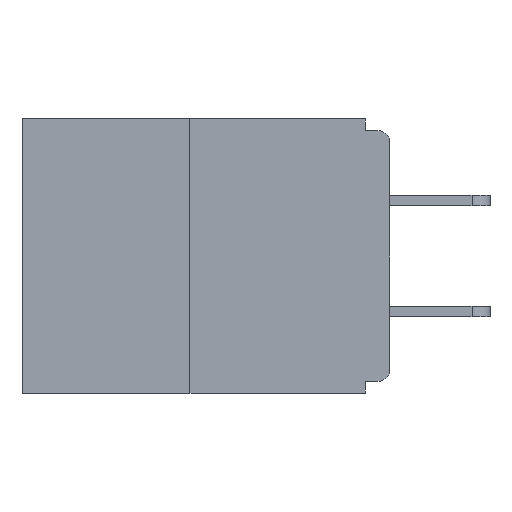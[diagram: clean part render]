
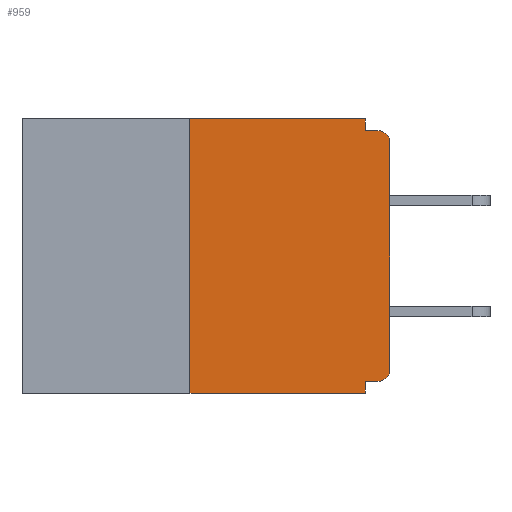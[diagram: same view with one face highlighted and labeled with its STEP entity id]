
A CAD part, left-side view. The second image highlights one B-rep face of the part: STEP entity #959.
In plain terms, the highlighted planar face has unit normal (-1, 0, 0).
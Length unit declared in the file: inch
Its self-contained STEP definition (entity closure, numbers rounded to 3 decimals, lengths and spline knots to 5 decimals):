
#425 = VECTOR ( 'NONE', #7176, 39.37008 ) ;
#959 = ADVANCED_FACE ( 'NONE', ( #2460 ), #17835, .F. ) ;
#1201 = VERTEX_POINT ( 'NONE', #17958 ) ;
#1491 = CARTESIAN_POINT ( 'NONE',  ( 0., 0.031, -0.015 ) ) ;
#1503 = VERTEX_POINT ( 'NONE', #8946 ) ;
#1510 = ORIENTED_EDGE ( 'NONE', *, *, #19461, .F. ) ;
#1680 = LINE ( 'NONE', #15199, #425 ) ;
#2442 = AXIS2_PLACEMENT_3D ( 'NONE', #6521, #6595, #19144 ) ;
#2460 = FACE_OUTER_BOUND ( 'NONE', #2973, .T. ) ;
#2553 = CARTESIAN_POINT ( 'NONE',  ( 0., 0.25, 0. ) ) ;
#2615 = CARTESIAN_POINT ( 'NONE',  ( 0., 0., -0.313 ) ) ;
#2715 = VECTOR ( 'NONE', #12299, 39.37008 ) ;
#2721 = EDGE_CURVE ( 'NONE', #8084, #14545, #8117, .T. ) ;
#2916 = CARTESIAN_POINT ( 'NONE',  ( 0., 0.031, 0. ) ) ;
#2940 = CARTESIAN_POINT ( 'NONE',  ( 0., 0.46, 0. ) ) ;
#2973 = EDGE_LOOP ( 'NONE', ( #14722, #11484, #11318, #6798, #1510, #3200, #17173, #15028, #7374, #11080 ) ) ;
#3147 = CARTESIAN_POINT ( 'NONE',  ( 0., 0.015, -0.328 ) ) ;
#3200 = ORIENTED_EDGE ( 'NONE', *, *, #8061, .T. ) ;
#3226 = CARTESIAN_POINT ( 'NONE',  ( 0., 0.015, -0.03 ) ) ;
#3694 = LINE ( 'NONE', #2940, #15866 ) ;
#4502 = CARTESIAN_POINT ( 'NONE',  ( 0., 0.031, -0.343 ) ) ;
#4614 = CARTESIAN_POINT ( 'NONE',  ( 0., 0.031, -0.343 ) ) ;
#4905 = EDGE_CURVE ( 'NONE', #20521, #1201, #19441, .T. ) ;
#5361 = CARTESIAN_POINT ( 'NONE',  ( 0., 0.46, -0.343 ) ) ;
#5876 = EDGE_CURVE ( 'NONE', #1201, #6665, #3694, .T. ) ;
#5906 = EDGE_CURVE ( 'NONE', #6817, #12715, #7424, .T. ) ;
#6147 = EDGE_CURVE ( 'NONE', #6665, #8084, #1680, .T. ) ;
#6521 = CARTESIAN_POINT ( 'NONE',  ( 0., 0.46, 0. ) ) ;
#6595 = DIRECTION ( 'NONE',  ( 1., 0., 0. ) ) ;
#6665 = VERTEX_POINT ( 'NONE', #2916 ) ;
#6798 = ORIENTED_EDGE ( 'NONE', *, *, #5906, .F. ) ;
#6817 = VERTEX_POINT ( 'NONE', #9434 ) ;
#7176 = DIRECTION ( 'NONE',  ( 0., 0., -1. ) ) ;
#7218 = LINE ( 'NONE', #7457, #2715 ) ;
#7374 = ORIENTED_EDGE ( 'NONE', *, *, #2721, .F. ) ;
#7424 = LINE ( 'NONE', #4614, #7663 ) ;
#7457 = CARTESIAN_POINT ( 'NONE',  ( 0., 0., 0. ) ) ;
#7663 = VECTOR ( 'NONE', #13121, 39.37008 ) ;
#7824 = EDGE_CURVE ( 'NONE', #20521, #12715, #13310, .T. ) ;
#8061 = EDGE_CURVE ( 'NONE', #15175, #11183, #15793, .T. ) ;
#8084 = VERTEX_POINT ( 'NONE', #1491 ) ;
#8117 = LINE ( 'NONE', #15813, #13808 ) ;
#8866 = EDGE_CURVE ( 'NONE', #1503, #14545, #14356, .T. ) ;
#8946 = CARTESIAN_POINT ( 'NONE',  ( 0., 0., -0.03 ) ) ;
#9434 = CARTESIAN_POINT ( 'NONE',  ( 0., 0.031, -0.328 ) ) ;
#11080 = ORIENTED_EDGE ( 'NONE', *, *, #6147, .F. ) ;
#11163 = AXIS2_PLACEMENT_3D ( 'NONE', #18859, #13949, #17351 ) ;
#11183 = VERTEX_POINT ( 'NONE', #2615 ) ;
#11219 = DIRECTION ( 'NONE',  ( -1., 0., 0. ) ) ;
#11318 = ORIENTED_EDGE ( 'NONE', *, *, #7824, .T. ) ;
#11467 = CARTESIAN_POINT ( 'NONE',  ( 0., 0.015, -0.015 ) ) ;
#11484 = ORIENTED_EDGE ( 'NONE', *, *, #4905, .F. ) ;
#11614 = DIRECTION ( 'NONE',  ( 0., -1., 0. ) ) ;
#11673 = CARTESIAN_POINT ( 'NONE',  ( 0., 0.25, -0.343 ) ) ;
#12299 = DIRECTION ( 'NONE',  ( 0., 0., 1. ) ) ;
#12368 = AXIS2_PLACEMENT_3D ( 'NONE', #3226, #11219, #17541 ) ;
#12590 = DIRECTION ( 'NONE',  ( 0., -1., 0. ) ) ;
#12621 = EDGE_CURVE ( 'NONE', #11183, #1503, #7218, .T. ) ;
#12715 = VERTEX_POINT ( 'NONE', #4502 ) ;
#13121 = DIRECTION ( 'NONE',  ( 0., 0., -1. ) ) ;
#13310 = LINE ( 'NONE', #5361, #17031 ) ;
#13808 = VECTOR ( 'NONE', #17337, 39.37008 ) ;
#13949 = DIRECTION ( 'NONE',  ( -1., 0., 0. ) ) ;
#14356 = CIRCLE ( 'NONE', #12368, 0.015 ) ;
#14545 = VERTEX_POINT ( 'NONE', #11467 ) ;
#14722 = ORIENTED_EDGE ( 'NONE', *, *, #5876, .F. ) ;
#15028 = ORIENTED_EDGE ( 'NONE', *, *, #8866, .T. ) ;
#15175 = VERTEX_POINT ( 'NONE', #3147 ) ;
#15199 = CARTESIAN_POINT ( 'NONE',  ( 0., 0.031, 0. ) ) ;
#15227 = VECTOR ( 'NONE', #16840, 39.37008 ) ;
#15793 = CIRCLE ( 'NONE', #11163, 0.015 ) ;
#15813 = CARTESIAN_POINT ( 'NONE',  ( 0., 0., -0.015 ) ) ;
#15866 = VECTOR ( 'NONE', #12590, 39.37008 ) ;
#16840 = DIRECTION ( 'NONE',  ( 0., 0., 1. ) ) ;
#17031 = VECTOR ( 'NONE', #11614, 39.37008 ) ;
#17091 = VECTOR ( 'NONE', #19131, 39.37008 ) ;
#17173 = ORIENTED_EDGE ( 'NONE', *, *, #12621, .T. ) ;
#17337 = DIRECTION ( 'NONE',  ( 0., -1., 0. ) ) ;
#17351 = DIRECTION ( 'NONE',  ( 0., 0., -1. ) ) ;
#17541 = DIRECTION ( 'NONE',  ( 0., 0., -1. ) ) ;
#17835 = PLANE ( 'NONE',  #2442 ) ;
#17958 = CARTESIAN_POINT ( 'NONE',  ( 0., 0.25, 0. ) ) ;
#18846 = CARTESIAN_POINT ( 'NONE',  ( 0., 0., -0.328 ) ) ;
#18859 = CARTESIAN_POINT ( 'NONE',  ( 0., 0.015, -0.313 ) ) ;
#19131 = DIRECTION ( 'NONE',  ( 0., 1., 0. ) ) ;
#19144 = DIRECTION ( 'NONE',  ( 0., 0., -1. ) ) ;
#19441 = LINE ( 'NONE', #2553, #15227 ) ;
#19461 = EDGE_CURVE ( 'NONE', #15175, #6817, #20334, .T. ) ;
#20334 = LINE ( 'NONE', #18846, #17091 ) ;
#20521 = VERTEX_POINT ( 'NONE', #11673 ) ;
